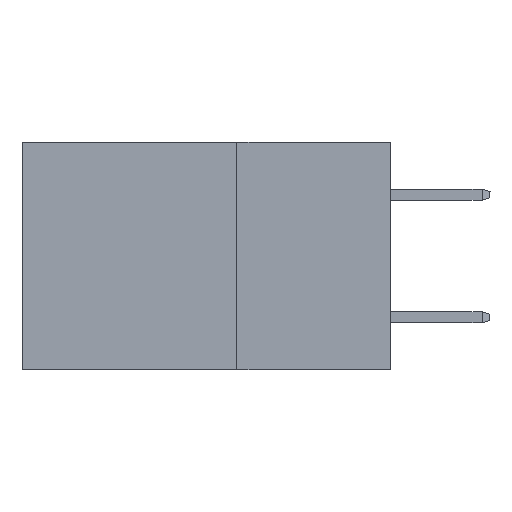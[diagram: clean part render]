
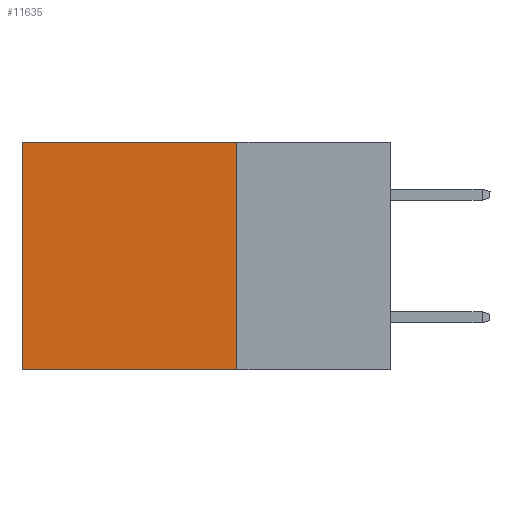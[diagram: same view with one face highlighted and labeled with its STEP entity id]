
A CAD part, left-side view. The second image highlights one B-rep face of the part: STEP entity #11635.
In plain terms, the highlighted planar face has unit normal (-1, 0, 0).
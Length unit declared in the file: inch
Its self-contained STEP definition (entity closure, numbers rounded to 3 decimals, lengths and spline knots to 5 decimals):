
#10 = VERTEX_POINT ( 'NONE', #1093 ) ;
#395 = ORIENTED_EDGE ( 'NONE', *, *, #2044, .F. ) ;
#670 = DIRECTION ( 'NONE',  ( 0., 0., -1. ) ) ;
#883 = CARTESIAN_POINT ( 'NONE',  ( 0.2875, 0.6, 0. ) ) ;
#1093 = CARTESIAN_POINT ( 'NONE',  ( 0.2875, 0.25, -0.37 ) ) ;
#2044 = EDGE_CURVE ( 'NONE', #10, #11363, #13834, .T. ) ;
#2146 = VECTOR ( 'NONE', #11498, 39.37008 ) ;
#2514 = ORIENTED_EDGE ( 'NONE', *, *, #11694, .F. ) ;
#3695 = VECTOR ( 'NONE', #9510, 39.37008 ) ;
#3739 = EDGE_CURVE ( 'NONE', #11721, #11363, #5074, .T. ) ;
#4973 = ORIENTED_EDGE ( 'NONE', *, *, #11591, .T. ) ;
#5074 = LINE ( 'NONE', #11292, #2146 ) ;
#6220 = LINE ( 'NONE', #7299, #3695 ) ;
#6222 = CARTESIAN_POINT ( 'NONE',  ( 0.2875, 0.25, 0. ) ) ;
#6556 = EDGE_LOOP ( 'NONE', ( #10095, #395, #2514, #4973 ) ) ;
#7141 = VECTOR ( 'NONE', #8721, 39.37008 ) ;
#7299 = CARTESIAN_POINT ( 'NONE',  ( 0.2875, 0.25, 0. ) ) ;
#7441 = DIRECTION ( 'NONE',  ( 1., 0., 0. ) ) ;
#7633 = VERTEX_POINT ( 'NONE', #6222 ) ;
#8185 = FACE_OUTER_BOUND ( 'NONE', #6556, .T. ) ;
#8721 = DIRECTION ( 'NONE',  ( 0., 0., -1. ) ) ;
#9063 = CARTESIAN_POINT ( 'NONE',  ( 0.2875, 0.6, -0.37 ) ) ;
#9510 = DIRECTION ( 'NONE',  ( 0., 1., 0. ) ) ;
#9589 = CARTESIAN_POINT ( 'NONE',  ( 0.2875, 0.25, 0. ) ) ;
#10095 = ORIENTED_EDGE ( 'NONE', *, *, #3739, .T. ) ;
#11073 = VECTOR ( 'NONE', #12661, 39.37008 ) ;
#11292 = CARTESIAN_POINT ( 'NONE',  ( 0.2875, 0.6, 0. ) ) ;
#11363 = VERTEX_POINT ( 'NONE', #9063 ) ;
#11498 = DIRECTION ( 'NONE',  ( 0., 0., -1. ) ) ;
#11591 = EDGE_CURVE ( 'NONE', #7633, #11721, #6220, .T. ) ;
#11635 = ADVANCED_FACE ( 'NONE', ( #8185 ), #12781, .F. ) ;
#11694 = EDGE_CURVE ( 'NONE', #7633, #10, #13166, .T. ) ;
#11721 = VERTEX_POINT ( 'NONE', #883 ) ;
#12631 = CARTESIAN_POINT ( 'NONE',  ( 0.2875, 0.25, -0.37 ) ) ;
#12661 = DIRECTION ( 'NONE',  ( 0., 1., 0. ) ) ;
#12781 = PLANE ( 'NONE',  #13342 ) ;
#13166 = LINE ( 'NONE', #13904, #7141 ) ;
#13342 = AXIS2_PLACEMENT_3D ( 'NONE', #9589, #7441, #670 ) ;
#13834 = LINE ( 'NONE', #12631, #11073 ) ;
#13904 = CARTESIAN_POINT ( 'NONE',  ( 0.2875, 0.25, 0. ) ) ;
